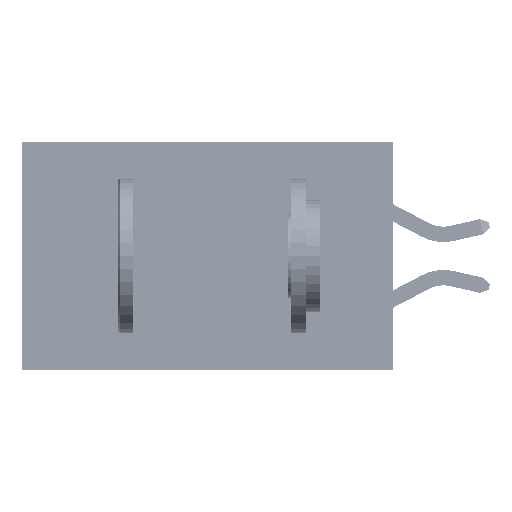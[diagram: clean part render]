
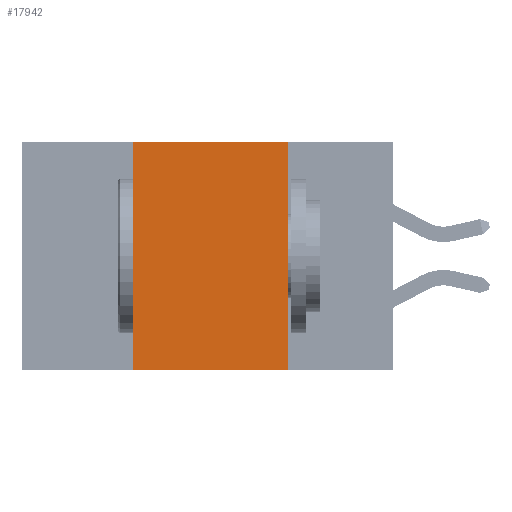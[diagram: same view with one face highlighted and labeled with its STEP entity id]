
A CAD part, left-side view. The second image highlights one B-rep face of the part: STEP entity #17942.
In plain terms, the highlighted planar face has unit normal (-1, 0, 0).
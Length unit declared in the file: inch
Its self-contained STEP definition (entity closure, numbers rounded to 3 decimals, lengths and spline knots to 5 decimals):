
#35 = CARTESIAN_POINT ( 'NONE',  ( 0., 0.6, 0. ) ) ;
#801 = CARTESIAN_POINT ( 'NONE',  ( 0., 0.42, -0.37 ) ) ;
#2709 = ORIENTED_EDGE ( 'NONE', *, *, #27992, .T. ) ;
#3428 = DIRECTION ( 'NONE',  ( 0., -1., 0. ) ) ;
#3977 = LINE ( 'NONE', #27708, #16726 ) ;
#4788 = CARTESIAN_POINT ( 'NONE',  ( 0., 0.42, 0. ) ) ;
#5027 = CARTESIAN_POINT ( 'NONE',  ( 0., 0.6, 0. ) ) ;
#5090 = DIRECTION ( 'NONE',  ( 0., 0., 1. ) ) ;
#5249 = CARTESIAN_POINT ( 'NONE',  ( 0., 0.42, 0. ) ) ;
#6554 = VERTEX_POINT ( 'NONE', #801 ) ;
#7678 = AXIS2_PLACEMENT_3D ( 'NONE', #5027, #10247, #33434 ) ;
#8431 = EDGE_CURVE ( 'NONE', #18619, #41801, #16169, .T. ) ;
#9551 = VERTEX_POINT ( 'NONE', #5249 ) ;
#10004 = DIRECTION ( 'NONE',  ( 0., -1., 0. ) ) ;
#10247 = DIRECTION ( 'NONE',  ( 1., 0., 0. ) ) ;
#14048 = ORIENTED_EDGE ( 'NONE', *, *, #21794, .F. ) ;
#15626 = VECTOR ( 'NONE', #3428, 39.37008 ) ;
#16169 = LINE ( 'NONE', #22460, #43238 ) ;
#16726 = VECTOR ( 'NONE', #10004, 39.37008 ) ;
#17942 = ADVANCED_FACE ( 'NONE', ( #33117 ), #31093, .F. ) ;
#18619 = VERTEX_POINT ( 'NONE', #39495 ) ;
#18715 = EDGE_LOOP ( 'NONE', ( #28721, #33487, #14048, #2709 ) ) ;
#21794 = EDGE_CURVE ( 'NONE', #6554, #9551, #26264, .T. ) ;
#22460 = CARTESIAN_POINT ( 'NONE',  ( 0., 0.17, 0. ) ) ;
#26098 = LINE ( 'NONE', #35, #15626 ) ;
#26264 = LINE ( 'NONE', #4788, #44540 ) ;
#27708 = CARTESIAN_POINT ( 'NONE',  ( 0., 0.6, -0.37 ) ) ;
#27992 = EDGE_CURVE ( 'NONE', #6554, #41801, #3977, .T. ) ;
#28721 = ORIENTED_EDGE ( 'NONE', *, *, #8431, .F. ) ;
#31093 = PLANE ( 'NONE',  #7678 ) ;
#33117 = FACE_OUTER_BOUND ( 'NONE', #18715, .T. ) ;
#33434 = DIRECTION ( 'NONE',  ( 0., 0., -1. ) ) ;
#33487 = ORIENTED_EDGE ( 'NONE', *, *, #44403, .F. ) ;
#38077 = CARTESIAN_POINT ( 'NONE',  ( 0., 0.17, -0.37 ) ) ;
#39495 = CARTESIAN_POINT ( 'NONE',  ( 0., 0.17, 0. ) ) ;
#41801 = VERTEX_POINT ( 'NONE', #38077 ) ;
#43238 = VECTOR ( 'NONE', #43929, 39.37008 ) ;
#43929 = DIRECTION ( 'NONE',  ( 0., 0., -1. ) ) ;
#44403 = EDGE_CURVE ( 'NONE', #9551, #18619, #26098, .T. ) ;
#44540 = VECTOR ( 'NONE', #5090, 39.37008 ) ;
